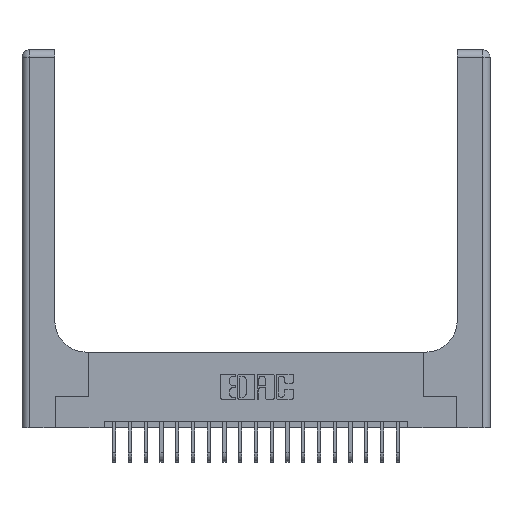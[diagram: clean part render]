
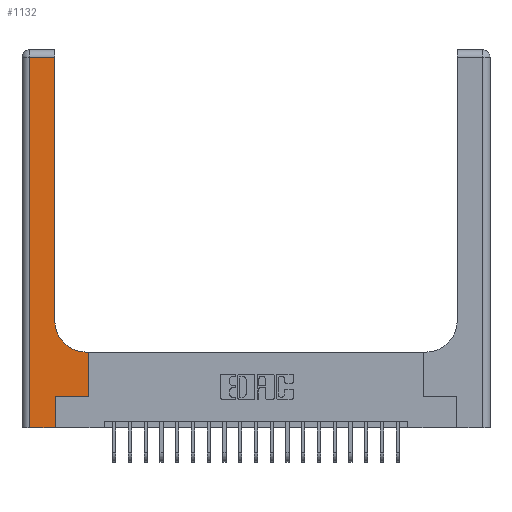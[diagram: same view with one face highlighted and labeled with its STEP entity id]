
A CAD part, top view. The second image highlights one B-rep face of the part: STEP entity #1132.
In plain terms, the highlighted planar face has unit normal (0, 0, 1).
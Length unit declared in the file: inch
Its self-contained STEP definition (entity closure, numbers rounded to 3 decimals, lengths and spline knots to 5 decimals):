
#373 = DIRECTION ( 'NONE',  ( -1., 0., 0. ) ) ;
#1132 = ADVANCED_FACE ( 'NONE', ( #3859 ), #11406, .F. ) ;
#1352 = EDGE_CURVE ( 'NONE', #5823, #2980, #8225, .T. ) ;
#1836 = VERTEX_POINT ( 'NONE', #2401 ) ;
#1961 = LINE ( 'NONE', #12642, #16621 ) ;
#1993 = CARTESIAN_POINT ( 'NONE',  ( 0.528, 0.25, 0.37 ) ) ;
#2401 = CARTESIAN_POINT ( 'NONE',  ( 0.26, 0.85, 0.37 ) ) ;
#2517 = LINE ( 'NONE', #19513, #13335 ) ;
#2707 = DIRECTION ( 'NONE',  ( 1., 0., 0. ) ) ;
#2980 = VERTEX_POINT ( 'NONE', #18626 ) ;
#3024 = ORIENTED_EDGE ( 'NONE', *, *, #1352, .T. ) ;
#3061 = EDGE_CURVE ( 'NONE', #21970, #14261, #11420, .T. ) ;
#3360 = EDGE_CURVE ( 'NONE', #2980, #18502, #10631, .T. ) ;
#3496 = ORIENTED_EDGE ( 'NONE', *, *, #7507, .T. ) ;
#3831 = CARTESIAN_POINT ( 'NONE',  ( 0.528, 0.25, 0.37 ) ) ;
#3859 = FACE_OUTER_BOUND ( 'NONE', #20783, .T. ) ;
#4678 = DIRECTION ( 'NONE',  ( 0., 1., 0. ) ) ;
#4685 = CARTESIAN_POINT ( 'NONE',  ( 0., 3., 0.37 ) ) ;
#5237 = ORIENTED_EDGE ( 'NONE', *, *, #8907, .T. ) ;
#5823 = VERTEX_POINT ( 'NONE', #21297 ) ;
#6025 = DIRECTION ( 'NONE',  ( 0., 0., -1. ) ) ;
#6302 = VECTOR ( 'NONE', #17291, 39.37008 ) ;
#6655 = CIRCLE ( 'NONE', #15114, 0.25 ) ;
#7215 = EDGE_CURVE ( 'NONE', #1836, #21970, #21590, .T. ) ;
#7507 = EDGE_CURVE ( 'NONE', #11999, #1836, #6655, .T. ) ;
#8174 = CARTESIAN_POINT ( 'NONE',  ( 0.26, 3., 0.37 ) ) ;
#8184 = CARTESIAN_POINT ( 'NONE',  ( 0., 0., 0.37 ) ) ;
#8225 = LINE ( 'NONE', #8184, #8480 ) ;
#8319 = CARTESIAN_POINT ( 'NONE',  ( 0.528, 0.6, 0.37 ) ) ;
#8480 = VECTOR ( 'NONE', #2707, 39.37008 ) ;
#8834 = EDGE_CURVE ( 'NONE', #14261, #5823, #1961, .T. ) ;
#8907 = EDGE_CURVE ( 'NONE', #10321, #11999, #2517, .T. ) ;
#9101 = ORIENTED_EDGE ( 'NONE', *, *, #3360, .T. ) ;
#9265 = EDGE_CURVE ( 'NONE', #18502, #15165, #10922, .T. ) ;
#10056 = VECTOR ( 'NONE', #12436, 39.37008 ) ;
#10152 = CARTESIAN_POINT ( 'NONE',  ( 0.265, 0.25, 0.37 ) ) ;
#10168 = CARTESIAN_POINT ( 'NONE',  ( 0.26, 2.94, 0.37 ) ) ;
#10321 = VERTEX_POINT ( 'NONE', #8319 ) ;
#10588 = CARTESIAN_POINT ( 'NONE',  ( 0.265, 0., 0.37 ) ) ;
#10631 = LINE ( 'NONE', #10588, #17685 ) ;
#10922 = LINE ( 'NONE', #10152, #6302 ) ;
#11016 = ORIENTED_EDGE ( 'NONE', *, *, #9265, .T. ) ;
#11406 = PLANE ( 'NONE',  #16786 ) ;
#11420 = LINE ( 'NONE', #20744, #21204 ) ;
#11999 = VERTEX_POINT ( 'NONE', #12433 ) ;
#12433 = CARTESIAN_POINT ( 'NONE',  ( 0.51, 0.6, 0.37 ) ) ;
#12436 = DIRECTION ( 'NONE',  ( 0., 1., 0. ) ) ;
#12480 = ORIENTED_EDGE ( 'NONE', *, *, #21567, .T. ) ;
#12600 = VECTOR ( 'NONE', #4678, 39.37008 ) ;
#12642 = CARTESIAN_POINT ( 'NONE',  ( 0.06, 3., 0.37 ) ) ;
#13335 = VECTOR ( 'NONE', #373, 39.37008 ) ;
#13431 = ORIENTED_EDGE ( 'NONE', *, *, #7215, .T. ) ;
#14261 = VERTEX_POINT ( 'NONE', #14928 ) ;
#14928 = CARTESIAN_POINT ( 'NONE',  ( 0.06, 2.94, 0.37 ) ) ;
#14931 = ORIENTED_EDGE ( 'NONE', *, *, #3061, .T. ) ;
#15114 = AXIS2_PLACEMENT_3D ( 'NONE', #21108, #15867, #19200 ) ;
#15165 = VERTEX_POINT ( 'NONE', #3831 ) ;
#15221 = ORIENTED_EDGE ( 'NONE', *, *, #8834, .T. ) ;
#15867 = DIRECTION ( 'NONE',  ( 0., 0., -1. ) ) ;
#16005 = DIRECTION ( 'NONE',  ( 0., -1., 0. ) ) ;
#16526 = DIRECTION ( 'NONE',  ( -1., 0., 0. ) ) ;
#16621 = VECTOR ( 'NONE', #16005, 39.37008 ) ;
#16786 = AXIS2_PLACEMENT_3D ( 'NONE', #4685, #6025, #16526 ) ;
#16857 = LINE ( 'NONE', #1993, #10056 ) ;
#17291 = DIRECTION ( 'NONE',  ( 1., 0., 0. ) ) ;
#17685 = VECTOR ( 'NONE', #21124, 39.37008 ) ;
#18502 = VERTEX_POINT ( 'NONE', #19692 ) ;
#18626 = CARTESIAN_POINT ( 'NONE',  ( 0.265, 0., 0.37 ) ) ;
#19200 = DIRECTION ( 'NONE',  ( 1., 0., 0. ) ) ;
#19513 = CARTESIAN_POINT ( 'NONE',  ( 0.26, 0.6, 0.37 ) ) ;
#19692 = CARTESIAN_POINT ( 'NONE',  ( 0.265, 0.25, 0.37 ) ) ;
#20744 = CARTESIAN_POINT ( 'NONE',  ( 0., 2.94, 0.37 ) ) ;
#20783 = EDGE_LOOP ( 'NONE', ( #13431, #14931, #15221, #3024, #9101, #11016, #12480, #5237, #3496 ) ) ;
#21055 = DIRECTION ( 'NONE',  ( -1., 0., 0. ) ) ;
#21108 = CARTESIAN_POINT ( 'NONE',  ( 0.51, 0.85, 0.37 ) ) ;
#21124 = DIRECTION ( 'NONE',  ( 0., 1., 0. ) ) ;
#21204 = VECTOR ( 'NONE', #21055, 39.37008 ) ;
#21297 = CARTESIAN_POINT ( 'NONE',  ( 0.06, 0., 0.37 ) ) ;
#21567 = EDGE_CURVE ( 'NONE', #15165, #10321, #16857, .T. ) ;
#21590 = LINE ( 'NONE', #8174, #12600 ) ;
#21970 = VERTEX_POINT ( 'NONE', #10168 ) ;
